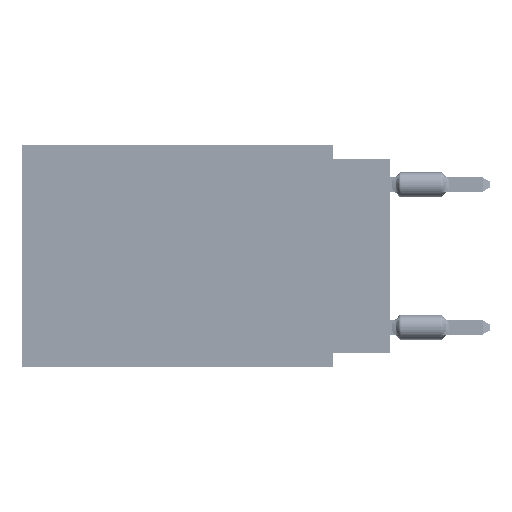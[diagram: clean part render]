
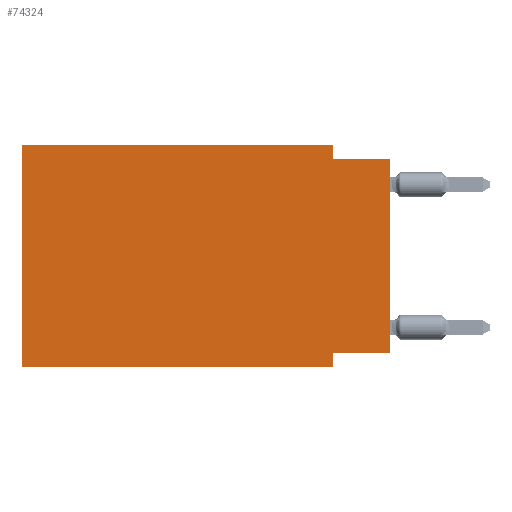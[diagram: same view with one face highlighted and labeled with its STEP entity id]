
A CAD part, left-side view. The second image highlights one B-rep face of the part: STEP entity #74324.
In plain terms, the highlighted planar face has unit normal (-1, 0, 0).
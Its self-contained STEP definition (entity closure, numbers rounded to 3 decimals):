
#184 = DIRECTION ( 'NONE',  ( 0., -1., 0. ) ) ;
#2163 = VECTOR ( 'NONE', #11745, 1000. ) ;
#3311 = VECTOR ( 'NONE', #30026, 1000. ) ;
#4296 = FACE_OUTER_BOUND ( 'NONE', #73461, .T. ) ;
#5181 = LINE ( 'NONE', #10880, #40117 ) ;
#5486 = DIRECTION ( 'NONE',  ( 0., 0., -1. ) ) ;
#5661 = DIRECTION ( 'NONE',  ( 0., 0., 1. ) ) ;
#6378 = VERTEX_POINT ( 'NONE', #18751 ) ;
#7856 = VERTEX_POINT ( 'NONE', #78878 ) ;
#8617 = DIRECTION ( 'NONE',  ( 0., 0., -1. ) ) ;
#10103 = CARTESIAN_POINT ( 'NONE',  ( 0., 0., 0. ) ) ;
#10880 = CARTESIAN_POINT ( 'NONE',  ( 0., 16.383, 0. ) ) ;
#11553 = CARTESIAN_POINT ( 'NONE',  ( 0., 0., -0.635 ) ) ;
#11745 = DIRECTION ( 'NONE',  ( 0., 1., 0. ) ) ;
#12587 = CARTESIAN_POINT ( 'NONE',  ( 0., 0., -0.635 ) ) ;
#13077 = LINE ( 'NONE', #24081, #75936 ) ;
#17111 = LINE ( 'NONE', #54176, #20181 ) ;
#17988 = AXIS2_PLACEMENT_3D ( 'NONE', #73061, #23787, #5486 ) ;
#18751 = CARTESIAN_POINT ( 'NONE',  ( 0., 2.54, -0.635 ) ) ;
#18820 = LINE ( 'NONE', #26545, #74835 ) ;
#20181 = VECTOR ( 'NONE', #36665, 1000. ) ;
#22850 = ORIENTED_EDGE ( 'NONE', *, *, #48137, .F. ) ;
#23445 = CARTESIAN_POINT ( 'NONE',  ( 0., 2.54, 0. ) ) ;
#23560 = ORIENTED_EDGE ( 'NONE', *, *, #59127, .F. ) ;
#23787 = DIRECTION ( 'NONE',  ( 1., 0., 0. ) ) ;
#24081 = CARTESIAN_POINT ( 'NONE',  ( 0., 2.54, 0. ) ) ;
#26046 = ORIENTED_EDGE ( 'NONE', *, *, #37221, .F. ) ;
#26545 = CARTESIAN_POINT ( 'NONE',  ( 0., 16.383, -9.906 ) ) ;
#27300 = VECTOR ( 'NONE', #5661, 1000. ) ;
#29668 = ORIENTED_EDGE ( 'NONE', *, *, #58876, .F. ) ;
#29674 = VERTEX_POINT ( 'NONE', #58968 ) ;
#30026 = DIRECTION ( 'NONE',  ( 0., 0., 1. ) ) ;
#33149 = VERTEX_POINT ( 'NONE', #54353 ) ;
#36134 = CARTESIAN_POINT ( 'NONE',  ( 0., 0., -9.271 ) ) ;
#36155 = LINE ( 'NONE', #10103, #3311 ) ;
#36665 = DIRECTION ( 'NONE',  ( 0., 0., -1. ) ) ;
#37221 = EDGE_CURVE ( 'NONE', #33149, #29674, #17111, .T. ) ;
#38017 = LINE ( 'NONE', #11553, #38244 ) ;
#38244 = VECTOR ( 'NONE', #184, 1000. ) ;
#40117 = VECTOR ( 'NONE', #54043, 1000. ) ;
#41900 = CARTESIAN_POINT ( 'NONE',  ( 0., 16.383, 0. ) ) ;
#42299 = ORIENTED_EDGE ( 'NONE', *, *, #67601, .F. ) ;
#44328 = VERTEX_POINT ( 'NONE', #12587 ) ;
#48137 = EDGE_CURVE ( 'NONE', #78149, #33149, #48808, .T. ) ;
#48808 = LINE ( 'NONE', #67512, #2163 ) ;
#52444 = CARTESIAN_POINT ( 'NONE',  ( 0., 16.383, -9.906 ) ) ;
#53643 = VERTEX_POINT ( 'NONE', #23445 ) ;
#54043 = DIRECTION ( 'NONE',  ( 0., -1., 0. ) ) ;
#54176 = CARTESIAN_POINT ( 'NONE',  ( 0., 2.54, -9.906 ) ) ;
#54353 = CARTESIAN_POINT ( 'NONE',  ( 0., 2.54, -9.271 ) ) ;
#58876 = EDGE_CURVE ( 'NONE', #53643, #6378, #13077, .T. ) ;
#58968 = CARTESIAN_POINT ( 'NONE',  ( 0., 2.54, -9.906 ) ) ;
#59127 = EDGE_CURVE ( 'NONE', #6378, #44328, #38017, .T. ) ;
#60446 = PLANE ( 'NONE',  #17988 ) ;
#60477 = EDGE_CURVE ( 'NONE', #73837, #29674, #18820, .T. ) ;
#62988 = ORIENTED_EDGE ( 'NONE', *, *, #73992, .F. ) ;
#63603 = DIRECTION ( 'NONE',  ( 0., -1., 0. ) ) ;
#67512 = CARTESIAN_POINT ( 'NONE',  ( 0., 0., -9.271 ) ) ;
#67519 = LINE ( 'NONE', #41900, #27300 ) ;
#67601 = EDGE_CURVE ( 'NONE', #73837, #7856, #67519, .T. ) ;
#70823 = ORIENTED_EDGE ( 'NONE', *, *, #71854, .T. ) ;
#71854 = EDGE_CURVE ( 'NONE', #78149, #44328, #36155, .T. ) ;
#73061 = CARTESIAN_POINT ( 'NONE',  ( 0., 16.383, 0. ) ) ;
#73461 = EDGE_LOOP ( 'NONE', ( #70823, #23560, #29668, #62988, #42299, #74141, #26046, #22850 ) ) ;
#73837 = VERTEX_POINT ( 'NONE', #52444 ) ;
#73992 = EDGE_CURVE ( 'NONE', #7856, #53643, #5181, .T. ) ;
#74141 = ORIENTED_EDGE ( 'NONE', *, *, #60477, .T. ) ;
#74324 = ADVANCED_FACE ( 'NONE', ( #4296 ), #60446, .F. ) ;
#74835 = VECTOR ( 'NONE', #63603, 1000. ) ;
#75936 = VECTOR ( 'NONE', #8617, 1000. ) ;
#78149 = VERTEX_POINT ( 'NONE', #36134 ) ;
#78878 = CARTESIAN_POINT ( 'NONE',  ( 0., 16.383, 0. ) ) ;
